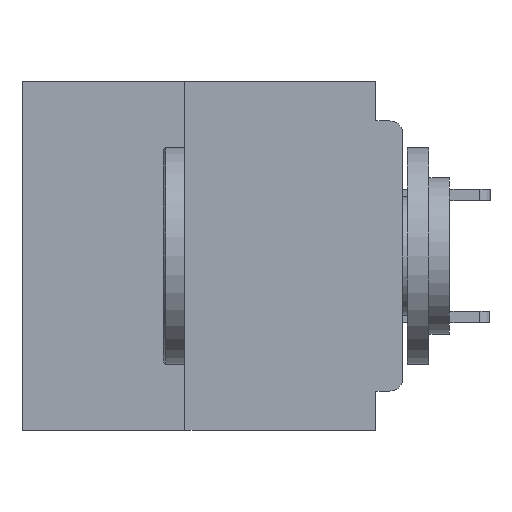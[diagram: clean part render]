
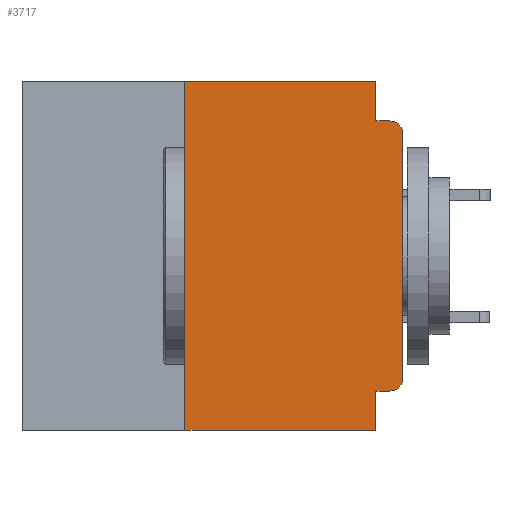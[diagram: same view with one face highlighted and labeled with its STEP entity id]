
A CAD part, left-side view. The second image highlights one B-rep face of the part: STEP entity #3717.
In plain terms, the highlighted planar face has unit normal (-1, 0, 0).
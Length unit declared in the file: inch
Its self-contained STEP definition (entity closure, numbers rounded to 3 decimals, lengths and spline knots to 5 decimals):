
#92 = CIRCLE ( 'NONE', #29163, 0.015 ) ;
#492 = CARTESIAN_POINT ( 'NONE',  ( 0., 0.031, -0.045 ) ) ;
#674 = VECTOR ( 'NONE', #37811, 39.37008 ) ;
#1174 = AXIS2_PLACEMENT_3D ( 'NONE', #43526, #42260, #42248 ) ;
#2970 = CARTESIAN_POINT ( 'NONE',  ( 0., 0.015, -0.34 ) ) ;
#3060 = CARTESIAN_POINT ( 'NONE',  ( 0., 0., -0.045 ) ) ;
#3370 = CARTESIAN_POINT ( 'NONE',  ( 0., 0.25, -0.4 ) ) ;
#3381 = CARTESIAN_POINT ( 'NONE',  ( 0., 0.031, 0. ) ) ;
#3717 = ADVANCED_FACE ( 'NONE', ( #26875 ), #42372, .F. ) ;
#3940 = CARTESIAN_POINT ( 'NONE',  ( 0., 0.031, -0.355 ) ) ;
#4715 = ORIENTED_EDGE ( 'NONE', *, *, #40888, .F. ) ;
#5553 = VECTOR ( 'NONE', #21055, 39.37008 ) ;
#5645 = DIRECTION ( 'NONE',  ( -1., 0., 0. ) ) ;
#6122 = CARTESIAN_POINT ( 'NONE',  ( 0., 0.015, -0.045 ) ) ;
#6847 = LINE ( 'NONE', #45515, #5553 ) ;
#7161 = DIRECTION ( 'NONE',  ( 0., 0., -1. ) ) ;
#10161 = VERTEX_POINT ( 'NONE', #38005 ) ;
#10921 = VECTOR ( 'NONE', #39851, 39.37008 ) ;
#12162 = VECTOR ( 'NONE', #24324, 39.37008 ) ;
#12170 = VERTEX_POINT ( 'NONE', #3370 ) ;
#12413 = EDGE_CURVE ( 'NONE', #12170, #39889, #17217, .T. ) ;
#12699 = VERTEX_POINT ( 'NONE', #44256 ) ;
#14767 = LINE ( 'NONE', #20238, #12162 ) ;
#15275 = EDGE_CURVE ( 'NONE', #10161, #16905, #92, .T. ) ;
#15731 = DIRECTION ( 'NONE',  ( 0., 0., -1. ) ) ;
#16212 = CARTESIAN_POINT ( 'NONE',  ( 0., 0., 0. ) ) ;
#16544 = EDGE_CURVE ( 'NONE', #39889, #43585, #43577, .T. ) ;
#16905 = VERTEX_POINT ( 'NONE', #44789 ) ;
#17217 = LINE ( 'NONE', #38388, #48389 ) ;
#18767 = EDGE_CURVE ( 'NONE', #16905, #41935, #25408, .T. ) ;
#20238 = CARTESIAN_POINT ( 'NONE',  ( 0., 0.031, -0.4 ) ) ;
#21055 = DIRECTION ( 'NONE',  ( 0., -1., 0. ) ) ;
#21710 = ORIENTED_EDGE ( 'NONE', *, *, #51644, .T. ) ;
#22639 = LINE ( 'NONE', #29607, #674 ) ;
#23542 = ORIENTED_EDGE ( 'NONE', *, *, #48049, .F. ) ;
#24101 = VECTOR ( 'NONE', #27719, 39.37008 ) ;
#24324 = DIRECTION ( 'NONE',  ( 0., 0., -1. ) ) ;
#25014 = CIRCLE ( 'NONE', #46117, 0.015 ) ;
#25188 = EDGE_CURVE ( 'NONE', #27936, #50880, #36254, .T. ) ;
#25408 = LINE ( 'NONE', #16212, #45852 ) ;
#26875 = FACE_OUTER_BOUND ( 'NONE', #38456, .T. ) ;
#27592 = ORIENTED_EDGE ( 'NONE', *, *, #31709, .T. ) ;
#27719 = DIRECTION ( 'NONE',  ( 0., -1., 0. ) ) ;
#27936 = VERTEX_POINT ( 'NONE', #492 ) ;
#28507 = DIRECTION ( 'NONE',  ( 0., 0., 1. ) ) ;
#28869 = EDGE_CURVE ( 'NONE', #43585, #27936, #45704, .T. ) ;
#28948 = ORIENTED_EDGE ( 'NONE', *, *, #16544, .F. ) ;
#29163 = AXIS2_PLACEMENT_3D ( 'NONE', #2970, #31737, #7161 ) ;
#29607 = CARTESIAN_POINT ( 'NONE',  ( 0., 0., -0.355 ) ) ;
#29628 = ORIENTED_EDGE ( 'NONE', *, *, #12413, .F. ) ;
#30240 = CARTESIAN_POINT ( 'NONE',  ( 0., 0.015, -0.06 ) ) ;
#31709 = EDGE_CURVE ( 'NONE', #41935, #50880, #25014, .T. ) ;
#31737 = DIRECTION ( 'NONE',  ( -1., 0., 0. ) ) ;
#31912 = CARTESIAN_POINT ( 'NONE',  ( 0., 0., -0.06 ) ) ;
#32770 = ORIENTED_EDGE ( 'NONE', *, *, #28869, .F. ) ;
#33578 = VECTOR ( 'NONE', #15731, 39.37008 ) ;
#34354 = DIRECTION ( 'NONE',  ( 0., 0., -1. ) ) ;
#34698 = CARTESIAN_POINT ( 'NONE',  ( 0., 0.25, 0. ) ) ;
#36254 = LINE ( 'NONE', #3060, #24101 ) ;
#36789 = VERTEX_POINT ( 'NONE', #3940 ) ;
#37490 = ORIENTED_EDGE ( 'NONE', *, *, #25188, .F. ) ;
#37811 = DIRECTION ( 'NONE',  ( 0., 1., 0. ) ) ;
#38005 = CARTESIAN_POINT ( 'NONE',  ( 0., 0.015, -0.355 ) ) ;
#38388 = CARTESIAN_POINT ( 'NONE',  ( 0., 0.25, -0.4 ) ) ;
#38456 = EDGE_LOOP ( 'NONE', ( #42792, #27592, #37490, #32770, #28948, #29628, #21710, #4715, #23542, #47964 ) ) ;
#39851 = DIRECTION ( 'NONE',  ( 0., -1., 0. ) ) ;
#39889 = VERTEX_POINT ( 'NONE', #34698 ) ;
#40888 = EDGE_CURVE ( 'NONE', #36789, #12699, #14767, .T. ) ;
#41935 = VERTEX_POINT ( 'NONE', #31912 ) ;
#42248 = DIRECTION ( 'NONE',  ( 0., 0., -1. ) ) ;
#42260 = DIRECTION ( 'NONE',  ( 1., 0., 0. ) ) ;
#42372 = PLANE ( 'NONE',  #1174 ) ;
#42514 = DIRECTION ( 'NONE',  ( 0., 0., 1. ) ) ;
#42792 = ORIENTED_EDGE ( 'NONE', *, *, #18767, .T. ) ;
#43526 = CARTESIAN_POINT ( 'NONE',  ( 0., 0.437, 0. ) ) ;
#43577 = LINE ( 'NONE', #43946, #10921 ) ;
#43585 = VERTEX_POINT ( 'NONE', #44120 ) ;
#43946 = CARTESIAN_POINT ( 'NONE',  ( 0., 0.437, 0. ) ) ;
#44120 = CARTESIAN_POINT ( 'NONE',  ( 0., 0.031, 0. ) ) ;
#44256 = CARTESIAN_POINT ( 'NONE',  ( 0., 0.031, -0.4 ) ) ;
#44789 = CARTESIAN_POINT ( 'NONE',  ( 0., 0., -0.34 ) ) ;
#45515 = CARTESIAN_POINT ( 'NONE',  ( 0., 0.437, -0.4 ) ) ;
#45704 = LINE ( 'NONE', #3381, #33578 ) ;
#45852 = VECTOR ( 'NONE', #28507, 39.37008 ) ;
#46117 = AXIS2_PLACEMENT_3D ( 'NONE', #30240, #5645, #34354 ) ;
#47964 = ORIENTED_EDGE ( 'NONE', *, *, #15275, .T. ) ;
#48049 = EDGE_CURVE ( 'NONE', #10161, #36789, #22639, .T. ) ;
#48389 = VECTOR ( 'NONE', #42514, 39.37008 ) ;
#50880 = VERTEX_POINT ( 'NONE', #6122 ) ;
#51644 = EDGE_CURVE ( 'NONE', #12170, #12699, #6847, .T. ) ;
